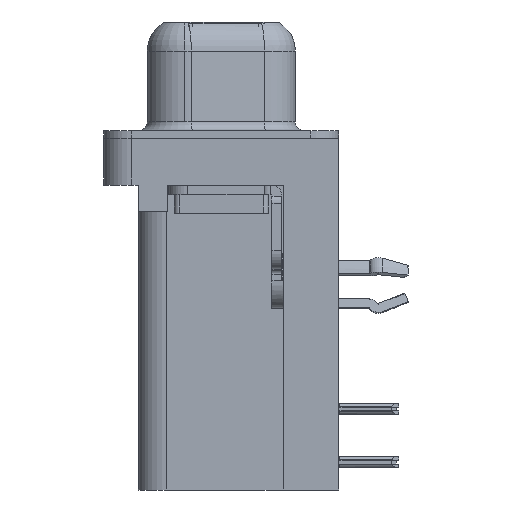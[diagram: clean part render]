
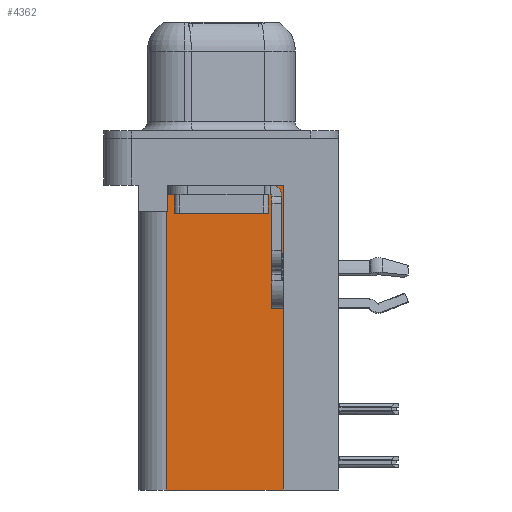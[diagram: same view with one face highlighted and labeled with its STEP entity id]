
A CAD part, left-side view. The second image highlights one B-rep face of the part: STEP entity #4362.
In plain terms, the highlighted planar face has unit normal (-1, 0, 0).
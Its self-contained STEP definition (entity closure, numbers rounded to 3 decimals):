
#1735 = VERTEX_POINT ( 'NONE', #33686 ) ;
#2367 = CARTESIAN_POINT ( 'NONE',  ( 3.79, 2.925, -18.76 ) ) ;
#3122 = DIRECTION ( 'NONE',  ( 0., 1., 0. ) ) ;
#3168 = DIRECTION ( 'NONE',  ( 1., 0., 0. ) ) ;
#4178 = VECTOR ( 'NONE', #30712, 1000. ) ;
#4362 = ADVANCED_FACE ( 'NONE', ( #4886 ), #6286, .F. ) ;
#4396 = LINE ( 'NONE', #27934, #4178 ) ;
#4437 = CARTESIAN_POINT ( 'NONE',  ( 3.79, -3.295, -18.76 ) ) ;
#4886 = FACE_OUTER_BOUND ( 'NONE', #35128, .T. ) ;
#5252 = CARTESIAN_POINT ( 'NONE',  ( 3.79, -3.295, -18.76 ) ) ;
#6286 = PLANE ( 'NONE',  #29091 ) ;
#7125 = CARTESIAN_POINT ( 'NONE',  ( 3.79, 2.925, -18.76 ) ) ;
#7139 = DIRECTION ( 'NONE',  ( 0., 1., 0. ) ) ;
#7337 = CARTESIAN_POINT ( 'NONE',  ( 3.79, 2.925, -3.9 ) ) ;
#7410 = CARTESIAN_POINT ( 'NONE',  ( 3.79, 0., -3.9 ) ) ;
#7889 = ORIENTED_EDGE ( 'NONE', *, *, #26982, .T. ) ;
#9484 = CARTESIAN_POINT ( 'NONE',  ( 3.79, 2.895, -2.5 ) ) ;
#10645 = ORIENTED_EDGE ( 'NONE', *, *, #22840, .T. ) ;
#11465 = ORIENTED_EDGE ( 'NONE', *, *, #15466, .T. ) ;
#12299 = VECTOR ( 'NONE', #19464, 1000. ) ;
#12480 = LINE ( 'NONE', #5252, #12299 ) ;
#12685 = VERTEX_POINT ( 'NONE', #9484 ) ;
#13089 = VERTEX_POINT ( 'NONE', #17255 ) ;
#13340 = EDGE_CURVE ( 'NONE', #1735, #16793, #12480, .T. ) ;
#15466 = EDGE_CURVE ( 'NONE', #1735, #31193, #25124, .T. ) ;
#15669 = CARTESIAN_POINT ( 'NONE',  ( 3.79, -3.295, -2.5 ) ) ;
#16061 = ORIENTED_EDGE ( 'NONE', *, *, #33495, .F. ) ;
#16793 = VERTEX_POINT ( 'NONE', #7125 ) ;
#17048 = VECTOR ( 'NONE', #24248, 1000. ) ;
#17177 = LINE ( 'NONE', #7410, #17048 ) ;
#17255 = CARTESIAN_POINT ( 'NONE',  ( 3.79, 2.895, -3.9 ) ) ;
#19015 = VECTOR ( 'NONE', #27413, 1000. ) ;
#19138 = VERTEX_POINT ( 'NONE', #7337 ) ;
#19191 = LINE ( 'NONE', #2367, #19015 ) ;
#19464 = DIRECTION ( 'NONE',  ( 0., 1., 0. ) ) ;
#19998 = EDGE_CURVE ( 'NONE', #31193, #12685, #20440, .T. ) ;
#20434 = VECTOR ( 'NONE', #7139, 1000. ) ;
#20440 = LINE ( 'NONE', #15669, #20434 ) ;
#22840 = EDGE_CURVE ( 'NONE', #12685, #13089, #4396, .T. ) ;
#24248 = DIRECTION ( 'NONE',  ( 0., 1., 0. ) ) ;
#25124 = LINE ( 'NONE', #33159, #25302 ) ;
#25302 = VECTOR ( 'NONE', #35703, 1000. ) ;
#25406 = CARTESIAN_POINT ( 'NONE',  ( 3.79, -3.295, -2.5 ) ) ;
#26982 = EDGE_CURVE ( 'NONE', #13089, #19138, #17177, .T. ) ;
#27413 = DIRECTION ( 'NONE',  ( 0., 0., 1. ) ) ;
#27934 = CARTESIAN_POINT ( 'NONE',  ( 3.79, 2.895, -3.9 ) ) ;
#29091 = AXIS2_PLACEMENT_3D ( 'NONE', #4437, #3168, #3122 ) ;
#30712 = DIRECTION ( 'NONE',  ( 0., 0., -1. ) ) ;
#31193 = VERTEX_POINT ( 'NONE', #25406 ) ;
#32000 = ORIENTED_EDGE ( 'NONE', *, *, #13340, .F. ) ;
#32677 = ORIENTED_EDGE ( 'NONE', *, *, #19998, .T. ) ;
#33159 = CARTESIAN_POINT ( 'NONE',  ( 3.79, -3.295, -18.76 ) ) ;
#33495 = EDGE_CURVE ( 'NONE', #16793, #19138, #19191, .T. ) ;
#33686 = CARTESIAN_POINT ( 'NONE',  ( 3.79, -3.295, -18.76 ) ) ;
#35128 = EDGE_LOOP ( 'NONE', ( #32677, #10645, #7889, #16061, #32000, #11465 ) ) ;
#35703 = DIRECTION ( 'NONE',  ( 0., 0., 1. ) ) ;
